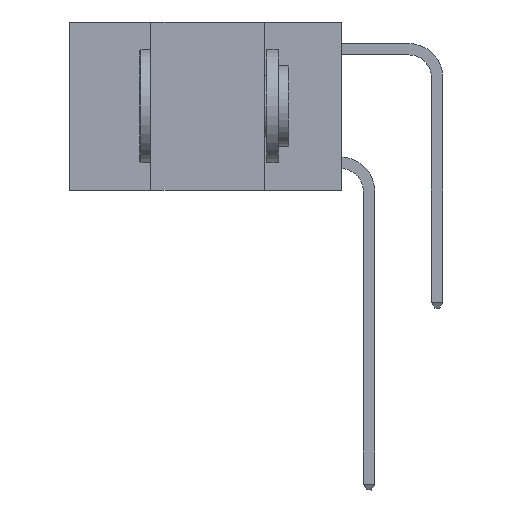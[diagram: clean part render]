
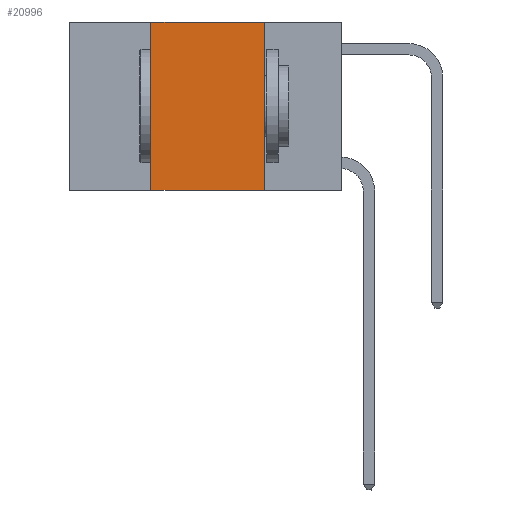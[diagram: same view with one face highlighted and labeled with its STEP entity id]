
A CAD part, left-side view. The second image highlights one B-rep face of the part: STEP entity #20996.
In plain terms, the highlighted planar face has unit normal (-1, 0, 0).
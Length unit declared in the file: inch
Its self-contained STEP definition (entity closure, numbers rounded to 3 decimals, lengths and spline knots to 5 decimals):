
#212 = VECTOR ( 'NONE', #4684, 39.37008 ) ;
#345 = DIRECTION ( 'NONE',  ( 1., 0., 0. ) ) ;
#1303 = CARTESIAN_POINT ( 'NONE',  ( 0., 0.42, -0.37 ) ) ;
#1446 = LINE ( 'NONE', #8186, #23640 ) ;
#4684 = DIRECTION ( 'NONE',  ( 0., 0., 1. ) ) ;
#5339 = CARTESIAN_POINT ( 'NONE',  ( 0., 0.42, 0. ) ) ;
#6028 = DIRECTION ( 'NONE',  ( 0., 0., -1. ) ) ;
#6199 = EDGE_LOOP ( 'NONE', ( #27566, #24910, #24350, #20603 ) ) ;
#6323 = CARTESIAN_POINT ( 'NONE',  ( 0., 0.17, -0.37 ) ) ;
#7810 = CARTESIAN_POINT ( 'NONE',  ( 0., 0.6, -0.37 ) ) ;
#8186 = CARTESIAN_POINT ( 'NONE',  ( 0., 0.17, 0. ) ) ;
#8420 = VERTEX_POINT ( 'NONE', #5339 ) ;
#9027 = VERTEX_POINT ( 'NONE', #20958 ) ;
#10577 = VECTOR ( 'NONE', #17029, 39.37008 ) ;
#10992 = CARTESIAN_POINT ( 'NONE',  ( 0., 0.42, 0. ) ) ;
#11571 = LINE ( 'NONE', #7810, #25836 ) ;
#13301 = EDGE_CURVE ( 'NONE', #8420, #9027, #18907, .T. ) ;
#14482 = AXIS2_PLACEMENT_3D ( 'NONE', #22039, #345, #15554 ) ;
#15405 = EDGE_CURVE ( 'NONE', #22868, #23763, #11571, .T. ) ;
#15554 = DIRECTION ( 'NONE',  ( 0., 0., -1. ) ) ;
#15581 = LINE ( 'NONE', #10992, #212 ) ;
#15693 = FACE_OUTER_BOUND ( 'NONE', #6199, .T. ) ;
#17029 = DIRECTION ( 'NONE',  ( 0., -1., 0. ) ) ;
#17175 = CARTESIAN_POINT ( 'NONE',  ( 0., 0.6, 0. ) ) ;
#17192 = EDGE_CURVE ( 'NONE', #22868, #8420, #15581, .T. ) ;
#18146 = PLANE ( 'NONE',  #14482 ) ;
#18907 = LINE ( 'NONE', #17175, #10577 ) ;
#19748 = EDGE_CURVE ( 'NONE', #9027, #23763, #1446, .T. ) ;
#20603 = ORIENTED_EDGE ( 'NONE', *, *, #15405, .T. ) ;
#20958 = CARTESIAN_POINT ( 'NONE',  ( 0., 0.17, 0. ) ) ;
#20996 = ADVANCED_FACE ( 'NONE', ( #15693 ), #18146, .F. ) ;
#22039 = CARTESIAN_POINT ( 'NONE',  ( 0., 0.6, 0. ) ) ;
#22868 = VERTEX_POINT ( 'NONE', #1303 ) ;
#23640 = VECTOR ( 'NONE', #6028, 39.37008 ) ;
#23763 = VERTEX_POINT ( 'NONE', #6323 ) ;
#24350 = ORIENTED_EDGE ( 'NONE', *, *, #17192, .F. ) ;
#24910 = ORIENTED_EDGE ( 'NONE', *, *, #13301, .F. ) ;
#25836 = VECTOR ( 'NONE', #26963, 39.37008 ) ;
#26963 = DIRECTION ( 'NONE',  ( 0., -1., 0. ) ) ;
#27566 = ORIENTED_EDGE ( 'NONE', *, *, #19748, .F. ) ;
